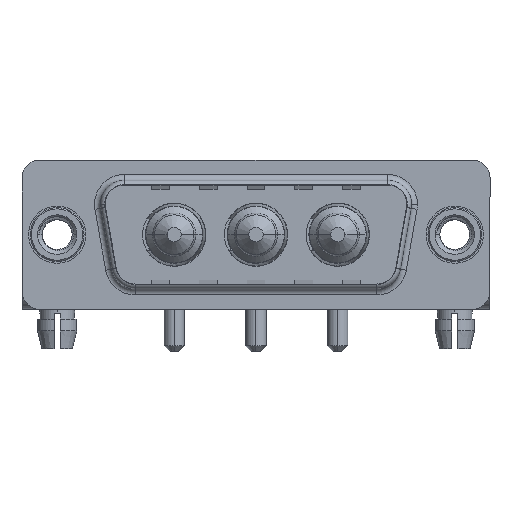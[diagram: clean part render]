
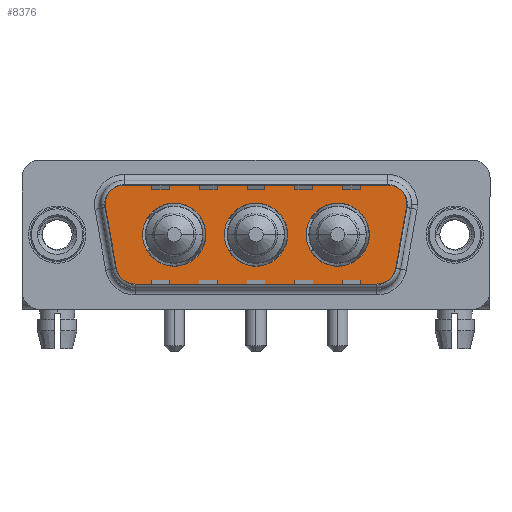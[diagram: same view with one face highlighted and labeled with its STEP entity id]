
A CAD part, top view. The second image highlights one B-rep face of the part: STEP entity #8376.
In plain terms, the highlighted planar face has unit normal (0, 0, 1).
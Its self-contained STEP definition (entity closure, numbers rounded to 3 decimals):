
#311 = CIRCLE ( 'NONE', #14597, 2.65 ) ;
#336 = VERTEX_POINT ( 'NONE', #12171 ) ;
#600 = DIRECTION ( 'NONE',  ( 0., 0., 1. ) ) ;
#851 = CIRCLE ( 'NONE', #10736, 2.65 ) ;
#1345 = CARTESIAN_POINT ( 'NONE',  ( 29.859, 2.553, 0. ) ) ;
#1349 = CARTESIAN_POINT ( 'NONE',  ( 27.889, 2.9, 0. ) ) ;
#1355 = DIRECTION ( 'NONE',  ( 0., 0., 1. ) ) ;
#1591 = DIRECTION ( 'NONE',  ( 1., 0., 0. ) ) ;
#1679 = CARTESIAN_POINT ( 'NONE',  ( 27.889, 2.9, 0. ) ) ;
#1681 = EDGE_CURVE ( 'NONE', #10867, #6459, #16814, .T. ) ;
#1911 = FACE_BOUND ( 'NONE', #3409, .T. ) ;
#2096 = DIRECTION ( 'NONE',  ( 0., 0., 1. ) ) ;
#2276 = EDGE_CURVE ( 'NONE', #2429, #336, #3828, .T. ) ;
#2310 = CARTESIAN_POINT ( 'NONE',  ( 6.434, -4.9, 0. ) ) ;
#2429 = VERTEX_POINT ( 'NONE', #16502 ) ;
#2564 = VERTEX_POINT ( 'NONE', #1345 ) ;
#2718 = EDGE_CURVE ( 'NONE', #2726, #12600, #311, .T. ) ;
#2726 = VERTEX_POINT ( 'NONE', #14660 ) ;
#3181 = EDGE_LOOP ( 'NONE', ( #14801, #3851, #4512, #16516, #7948, #13944, #10413, #15232, #6264 ) ) ;
#3195 = FACE_OUTER_BOUND ( 'NONE', #3181, .T. ) ;
#3287 = DIRECTION ( 'NONE',  ( 0., 0., 1. ) ) ;
#3389 = LINE ( 'NONE', #13885, #5990 ) ;
#3409 = EDGE_LOOP ( 'NONE', ( #14097, #16558 ) ) ;
#3475 = EDGE_LOOP ( 'NONE', ( #14630, #13750 ) ) ;
#3765 = VECTOR ( 'NONE', #12125, 1000. ) ;
#3828 = CIRCLE ( 'NONE', #5477, 2.65 ) ;
#3851 = ORIENTED_EDGE ( 'NONE', *, *, #11889, .T. ) ;
#3912 = DIRECTION ( 'NONE',  ( 1., 0., 0. ) ) ;
#4164 = VERTEX_POINT ( 'NONE', #9484 ) ;
#4176 = DIRECTION ( 'NONE',  ( 1., 0., 0. ) ) ;
#4352 = DIRECTION ( 'NONE',  ( 1., 0., 0. ) ) ;
#4379 = EDGE_CURVE ( 'NONE', #16594, #10867, #8459, .T. ) ;
#4423 = DIRECTION ( 'NONE',  ( 1., 0., 0. ) ) ;
#4456 = CARTESIAN_POINT ( 'NONE',  ( 6.434, -4.9, 0. ) ) ;
#4512 = ORIENTED_EDGE ( 'NONE', *, *, #6104, .T. ) ;
#4631 = AXIS2_PLACEMENT_3D ( 'NONE', #14325, #10640, #3912 ) ;
#4747 = EDGE_CURVE ( 'NONE', #4164, #16129, #851, .T. ) ;
#4843 = CARTESIAN_POINT ( 'NONE',  ( 26.866, -4.9, 0. ) ) ;
#4967 = ORIENTED_EDGE ( 'NONE', *, *, #14607, .F. ) ;
#5018 = DIRECTION ( 'NONE',  ( 0.174, -0.985, 0. ) ) ;
#5033 = ORIENTED_EDGE ( 'NONE', *, *, #2276, .F. ) ;
#5162 = CIRCLE ( 'NONE', #14792, 2.65 ) ;
#5477 = AXIS2_PLACEMENT_3D ( 'NONE', #13308, #12198, #4352 ) ;
#5990 = VECTOR ( 'NONE', #13800, 1000. ) ;
#6104 = EDGE_CURVE ( 'NONE', #2564, #14855, #15134, .T. ) ;
#6135 = DIRECTION ( 'NONE',  ( 0., 0., 1. ) ) ;
#6264 = ORIENTED_EDGE ( 'NONE', *, *, #7932, .T. ) ;
#6277 = CIRCLE ( 'NONE', #4631, 2.65 ) ;
#6373 = CARTESIAN_POINT ( 'NONE',  ( 5.411, 4.9, 0. ) ) ;
#6415 = CARTESIAN_POINT ( 'NONE',  ( 26.866, -2.9, 0. ) ) ;
#6459 = VERTEX_POINT ( 'NONE', #13982 ) ;
#6707 = AXIS2_PLACEMENT_3D ( 'NONE', #6415, #1355, #4176 ) ;
#6917 = DIRECTION ( 'NONE',  ( -1., 0., 0. ) ) ;
#6991 = DIRECTION ( 'NONE',  ( 0., 0., 1. ) ) ;
#7151 = FACE_BOUND ( 'NONE', #9109, .T. ) ;
#7278 = VECTOR ( 'NONE', #12824, 1000. ) ;
#7669 = CARTESIAN_POINT ( 'NONE',  ( 27.889, 4.9, 0. ) ) ;
#7788 = CARTESIAN_POINT ( 'NONE',  ( 28.836, -3.247, 0. ) ) ;
#7870 = DIRECTION ( 'NONE',  ( -1., 0., 0. ) ) ;
#7932 = EDGE_CURVE ( 'NONE', #11902, #11148, #14104, .T. ) ;
#7948 = ORIENTED_EDGE ( 'NONE', *, *, #13076, .T. ) ;
#8376 = ADVANCED_FACE ( 'NONE', ( #1911, #7151, #15349, #3195 ), #13786, .T. ) ;
#8442 = CARTESIAN_POINT ( 'NONE',  ( 26.866, -2.9, 0. ) ) ;
#8459 = CIRCLE ( 'NONE', #14638, 2. ) ;
#8995 = EDGE_CURVE ( 'NONE', #11148, #15711, #14145, .T. ) ;
#9055 = CIRCLE ( 'NONE', #13181, 2. ) ;
#9109 = EDGE_LOOP ( 'NONE', ( #4967, #5033 ) ) ;
#9423 = CARTESIAN_POINT ( 'NONE',  ( 9.8, 0., 0. ) ) ;
#9438 = CARTESIAN_POINT ( 'NONE',  ( 7.15, 0., 0. ) ) ;
#9484 = CARTESIAN_POINT ( 'NONE',  ( 14., 0., 0. ) ) ;
#9593 = CARTESIAN_POINT ( 'NONE',  ( 16.65, 0., 0. ) ) ;
#9686 = DIRECTION ( 'NONE',  ( 0., 0., 1. ) ) ;
#9861 = CARTESIAN_POINT ( 'NONE',  ( 23.5, 0., 0. ) ) ;
#9911 = AXIS2_PLACEMENT_3D ( 'NONE', #1679, #9686, #6917 ) ;
#10175 = VECTOR ( 'NONE', #5018, 1000. ) ;
#10413 = ORIENTED_EDGE ( 'NONE', *, *, #1681, .T. ) ;
#10640 = DIRECTION ( 'NONE',  ( 0., 0., 1. ) ) ;
#10711 = CARTESIAN_POINT ( 'NONE',  ( 29.889, 2.9, 0. ) ) ;
#10736 = AXIS2_PLACEMENT_3D ( 'NONE', #9593, #6991, #4423 ) ;
#10867 = VERTEX_POINT ( 'NONE', #15956 ) ;
#11148 = VERTEX_POINT ( 'NONE', #4843 ) ;
#11295 = CIRCLE ( 'NONE', #17002, 2.65 ) ;
#11304 = VERTEX_POINT ( 'NONE', #7669 ) ;
#11480 = DIRECTION ( 'NONE',  ( 1., 0., 0. ) ) ;
#11580 = CARTESIAN_POINT ( 'NONE',  ( 3.441, 2.553, 0. ) ) ;
#11889 = EDGE_CURVE ( 'NONE', #15711, #2564, #13752, .T. ) ;
#11902 = VERTEX_POINT ( 'NONE', #4456 ) ;
#12125 = DIRECTION ( 'NONE',  ( 0.174, 0.985, 0. ) ) ;
#12171 = CARTESIAN_POINT ( 'NONE',  ( 26.15, 0., 0. ) ) ;
#12198 = DIRECTION ( 'NONE',  ( 0., 0., 1. ) ) ;
#12390 = DIRECTION ( 'NONE',  ( 1., 0., 0. ) ) ;
#12600 = VERTEX_POINT ( 'NONE', #9438 ) ;
#12638 = DIRECTION ( 'NONE',  ( 0., 0., 1. ) ) ;
#12795 = EDGE_CURVE ( 'NONE', #16129, #4164, #6277, .T. ) ;
#12824 = DIRECTION ( 'NONE',  ( 1., 0., 0. ) ) ;
#13045 = DIRECTION ( 'NONE',  ( 0., 0., 1. ) ) ;
#13076 = EDGE_CURVE ( 'NONE', #11304, #16594, #3389, .T. ) ;
#13087 = EDGE_CURVE ( 'NONE', #12600, #2726, #5162, .T. ) ;
#13181 = AXIS2_PLACEMENT_3D ( 'NONE', #15219, #12638, #13830 ) ;
#13308 = CARTESIAN_POINT ( 'NONE',  ( 23.5, 0., 0. ) ) ;
#13663 = CARTESIAN_POINT ( 'NONE',  ( 29.859, 2.553, 0. ) ) ;
#13750 = ORIENTED_EDGE ( 'NONE', *, *, #13087, .F. ) ;
#13752 = LINE ( 'NONE', #13663, #3765 ) ;
#13786 = PLANE ( 'NONE',  #15255 ) ;
#13800 = DIRECTION ( 'NONE',  ( -1., 0., 0. ) ) ;
#13830 = DIRECTION ( 'NONE',  ( -1., 0., 0. ) ) ;
#13885 = CARTESIAN_POINT ( 'NONE',  ( 5.411, 4.9, 0. ) ) ;
#13893 = DIRECTION ( 'NONE',  ( 1., 0., 0. ) ) ;
#13944 = ORIENTED_EDGE ( 'NONE', *, *, #4379, .T. ) ;
#13973 = CARTESIAN_POINT ( 'NONE',  ( 9.8, 0., 0. ) ) ;
#13982 = CARTESIAN_POINT ( 'NONE',  ( 4.464, -3.247, 0. ) ) ;
#14097 = ORIENTED_EDGE ( 'NONE', *, *, #12795, .F. ) ;
#14104 = LINE ( 'NONE', #2310, #7278 ) ;
#14145 = CIRCLE ( 'NONE', #6707, 2. ) ;
#14245 = AXIS2_PLACEMENT_3D ( 'NONE', #1349, #13045, #7870 ) ;
#14325 = CARTESIAN_POINT ( 'NONE',  ( 16.65, 0., 0. ) ) ;
#14472 = EDGE_CURVE ( 'NONE', #14855, #11304, #15938, .T. ) ;
#14597 = AXIS2_PLACEMENT_3D ( 'NONE', #9423, #16130, #1591 ) ;
#14607 = EDGE_CURVE ( 'NONE', #336, #2429, #11295, .T. ) ;
#14630 = ORIENTED_EDGE ( 'NONE', *, *, #2718, .F. ) ;
#14638 = AXIS2_PLACEMENT_3D ( 'NONE', #16173, #600, #12390 ) ;
#14660 = CARTESIAN_POINT ( 'NONE',  ( 12.45, 0., 0. ) ) ;
#14792 = AXIS2_PLACEMENT_3D ( 'NONE', #13973, #6135, #15362 ) ;
#14801 = ORIENTED_EDGE ( 'NONE', *, *, #8995, .T. ) ;
#14855 = VERTEX_POINT ( 'NONE', #10711 ) ;
#15134 = CIRCLE ( 'NONE', #14245, 2. ) ;
#15219 = CARTESIAN_POINT ( 'NONE',  ( 6.434, -2.9, 0. ) ) ;
#15232 = ORIENTED_EDGE ( 'NONE', *, *, #15655, .T. ) ;
#15255 = AXIS2_PLACEMENT_3D ( 'NONE', #8442, #3287, #11480 ) ;
#15349 = FACE_BOUND ( 'NONE', #3475, .T. ) ;
#15362 = DIRECTION ( 'NONE',  ( 1., 0., 0. ) ) ;
#15655 = EDGE_CURVE ( 'NONE', #6459, #11902, #9055, .T. ) ;
#15711 = VERTEX_POINT ( 'NONE', #7788 ) ;
#15938 = CIRCLE ( 'NONE', #9911, 2. ) ;
#15956 = CARTESIAN_POINT ( 'NONE',  ( 3.441, 2.553, 0. ) ) ;
#16129 = VERTEX_POINT ( 'NONE', #16824 ) ;
#16130 = DIRECTION ( 'NONE',  ( 0., 0., 1. ) ) ;
#16173 = CARTESIAN_POINT ( 'NONE',  ( 5.411, 2.9, 0. ) ) ;
#16502 = CARTESIAN_POINT ( 'NONE',  ( 20.85, 0., 0. ) ) ;
#16516 = ORIENTED_EDGE ( 'NONE', *, *, #14472, .T. ) ;
#16558 = ORIENTED_EDGE ( 'NONE', *, *, #4747, .F. ) ;
#16594 = VERTEX_POINT ( 'NONE', #6373 ) ;
#16814 = LINE ( 'NONE', #11580, #10175 ) ;
#16824 = CARTESIAN_POINT ( 'NONE',  ( 19.3, 0., 0. ) ) ;
#17002 = AXIS2_PLACEMENT_3D ( 'NONE', #9861, #2096, #13893 ) ;
